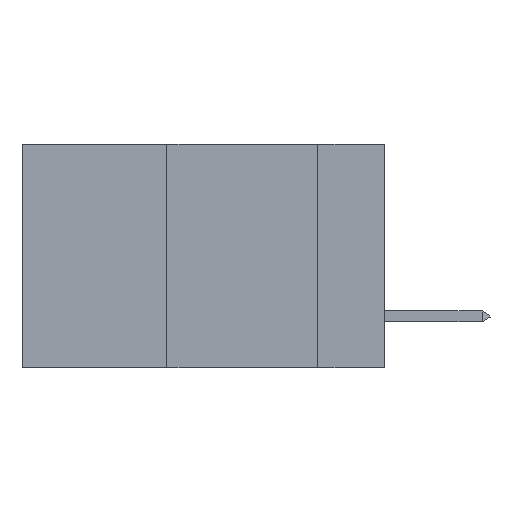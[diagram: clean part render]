
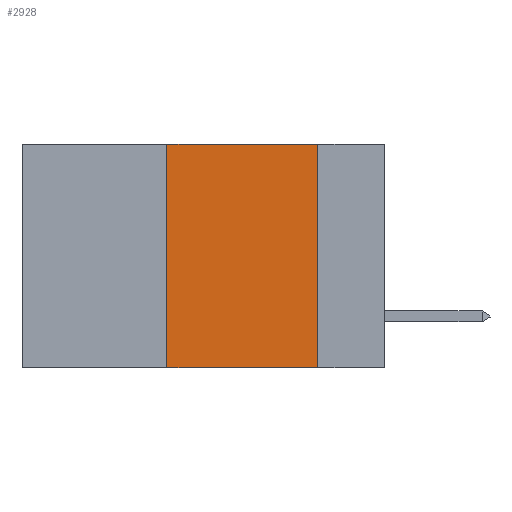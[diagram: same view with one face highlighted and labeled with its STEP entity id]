
A CAD part, left-side view. The second image highlights one B-rep face of the part: STEP entity #2928.
In plain terms, the highlighted planar face has unit normal (-1, 0, 0).
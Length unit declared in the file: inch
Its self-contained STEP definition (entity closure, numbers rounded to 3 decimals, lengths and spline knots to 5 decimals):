
#195 = ORIENTED_EDGE ( 'NONE', *, *, #5424, .T. ) ;
#586 = CARTESIAN_POINT ( 'NONE',  ( 0., 0.36, 0. ) ) ;
#624 = CARTESIAN_POINT ( 'NONE',  ( 0., 0.6, -0.37 ) ) ;
#839 = LINE ( 'NONE', #6593, #11631 ) ;
#1010 = VECTOR ( 'NONE', #13277, 39.37008 ) ;
#2483 = AXIS2_PLACEMENT_3D ( 'NONE', #5492, #11781, #5304 ) ;
#2928 = ADVANCED_FACE ( 'NONE', ( #8791 ), #7625, .F. ) ;
#3217 = CARTESIAN_POINT ( 'NONE',  ( 0., 0.11, 0. ) ) ;
#3395 = CARTESIAN_POINT ( 'NONE',  ( 0., 0.36, -0.37 ) ) ;
#4509 = CARTESIAN_POINT ( 'NONE',  ( 0., 0.6, 0. ) ) ;
#4678 = CARTESIAN_POINT ( 'NONE',  ( 0., 0.36, 0. ) ) ;
#5107 = EDGE_CURVE ( 'NONE', #10301, #13032, #13457, .T. ) ;
#5218 = LINE ( 'NONE', #4509, #13282 ) ;
#5304 = DIRECTION ( 'NONE',  ( 0., 0., -1. ) ) ;
#5424 = EDGE_CURVE ( 'NONE', #10301, #9463, #6735, .T. ) ;
#5492 = CARTESIAN_POINT ( 'NONE',  ( 0., 0.6, 0. ) ) ;
#5972 = DIRECTION ( 'NONE',  ( 0., -1., 0. ) ) ;
#6593 = CARTESIAN_POINT ( 'NONE',  ( 0., 0.11, 0. ) ) ;
#6735 = LINE ( 'NONE', #624, #8071 ) ;
#6737 = ORIENTED_EDGE ( 'NONE', *, *, #5107, .F. ) ;
#6794 = EDGE_LOOP ( 'NONE', ( #12085, #13838, #6737, #195 ) ) ;
#7625 = PLANE ( 'NONE',  #2483 ) ;
#7937 = VERTEX_POINT ( 'NONE', #3217 ) ;
#8071 = VECTOR ( 'NONE', #5972, 39.37008 ) ;
#8791 = FACE_OUTER_BOUND ( 'NONE', #6794, .T. ) ;
#8795 = DIRECTION ( 'NONE',  ( 0., 0., -1. ) ) ;
#9463 = VERTEX_POINT ( 'NONE', #12477 ) ;
#10090 = DIRECTION ( 'NONE',  ( 0., -1., 0. ) ) ;
#10301 = VERTEX_POINT ( 'NONE', #3395 ) ;
#11631 = VECTOR ( 'NONE', #8795, 39.37008 ) ;
#11781 = DIRECTION ( 'NONE',  ( 1., 0., 0. ) ) ;
#12085 = ORIENTED_EDGE ( 'NONE', *, *, #13331, .F. ) ;
#12477 = CARTESIAN_POINT ( 'NONE',  ( 0., 0.11, -0.37 ) ) ;
#13032 = VERTEX_POINT ( 'NONE', #586 ) ;
#13277 = DIRECTION ( 'NONE',  ( 0., 0., 1. ) ) ;
#13282 = VECTOR ( 'NONE', #10090, 39.37008 ) ;
#13331 = EDGE_CURVE ( 'NONE', #7937, #9463, #839, .T. ) ;
#13457 = LINE ( 'NONE', #4678, #1010 ) ;
#13688 = EDGE_CURVE ( 'NONE', #13032, #7937, #5218, .T. ) ;
#13838 = ORIENTED_EDGE ( 'NONE', *, *, #13688, .F. ) ;
